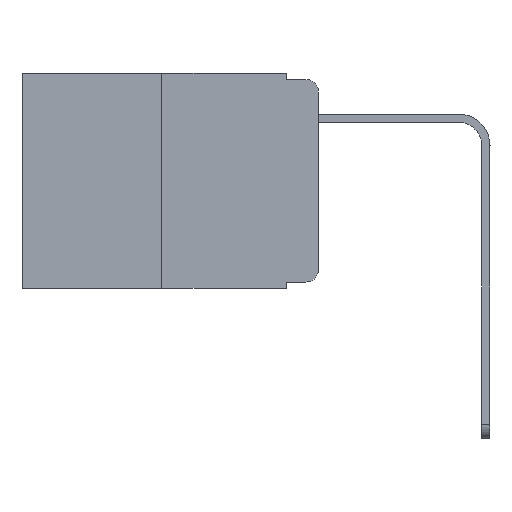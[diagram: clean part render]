
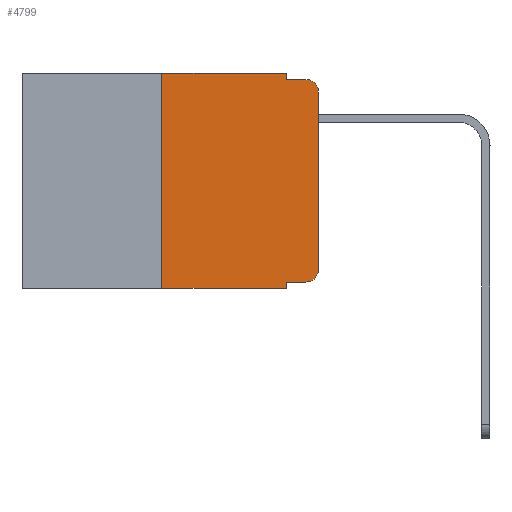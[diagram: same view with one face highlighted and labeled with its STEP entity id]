
A CAD part, left-side view. The second image highlights one B-rep face of the part: STEP entity #4799.
In plain terms, the highlighted planar face has unit normal (-1, 0, 0).
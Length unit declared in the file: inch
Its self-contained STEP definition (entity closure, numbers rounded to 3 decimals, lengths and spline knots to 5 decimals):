
#26 = VECTOR ( 'NONE', #664, 39.37008 ) ;
#181 = LINE ( 'NONE', #2816, #5194 ) ;
#367 = ORIENTED_EDGE ( 'NONE', *, *, #5825, .T. ) ;
#458 = CARTESIAN_POINT ( 'NONE',  ( 0., 0.473, 0. ) ) ;
#626 = EDGE_CURVE ( 'NONE', #7252, #5848, #4277, .T. ) ;
#664 = DIRECTION ( 'NONE',  ( 0., 0., 1. ) ) ;
#673 = CARTESIAN_POINT ( 'NONE',  ( 0., 0.02, -0.03 ) ) ;
#849 = VECTOR ( 'NONE', #5323, 39.37008 ) ;
#954 = ORIENTED_EDGE ( 'NONE', *, *, #626, .F. ) ;
#1013 = VECTOR ( 'NONE', #5104, 39.37008 ) ;
#1018 = VECTOR ( 'NONE', #8433, 39.37008 ) ;
#1101 = LINE ( 'NONE', #2845, #849 ) ;
#1261 = PLANE ( 'NONE',  #10363 ) ;
#1367 = EDGE_CURVE ( 'NONE', #1961, #3718, #2399, .T. ) ;
#1424 = EDGE_CURVE ( 'NONE', #5848, #6477, #9442, .T. ) ;
#1568 = CARTESIAN_POINT ( 'NONE',  ( 0., 0.25, 0. ) ) ;
#1750 = DIRECTION ( 'NONE',  ( 0., -1., 0. ) ) ;
#1810 = CARTESIAN_POINT ( 'NONE',  ( 0., 0.051, -0.01 ) ) ;
#1961 = VERTEX_POINT ( 'NONE', #6617 ) ;
#2343 = VECTOR ( 'NONE', #5141, 39.37008 ) ;
#2399 = LINE ( 'NONE', #1810, #5044 ) ;
#2476 = DIRECTION ( 'NONE',  ( -1., 0., 0. ) ) ;
#2496 = CIRCLE ( 'NONE', #4143, 0.02 ) ;
#2742 = DIRECTION ( 'NONE',  ( 0., 0., -1. ) ) ;
#2808 = CARTESIAN_POINT ( 'NONE',  ( 0., 0.473, 0. ) ) ;
#2816 = CARTESIAN_POINT ( 'NONE',  ( 0., 0.051, 0. ) ) ;
#2845 = CARTESIAN_POINT ( 'NONE',  ( 0., 0.051, -0.333 ) ) ;
#2861 = ORIENTED_EDGE ( 'NONE', *, *, #3949, .F. ) ;
#3322 = ORIENTED_EDGE ( 'NONE', *, *, #5238, .T. ) ;
#3520 = DIRECTION ( 'NONE',  ( 0., 0., -1. ) ) ;
#3547 = CARTESIAN_POINT ( 'NONE',  ( 0., 0., -0.313 ) ) ;
#3718 = VERTEX_POINT ( 'NONE', #6974 ) ;
#3790 = EDGE_CURVE ( 'NONE', #9570, #6513, #1101, .T. ) ;
#3949 = EDGE_CURVE ( 'NONE', #6477, #1961, #10287, .T. ) ;
#4033 = CARTESIAN_POINT ( 'NONE',  ( 0., 0.02, -0.333 ) ) ;
#4143 = AXIS2_PLACEMENT_3D ( 'NONE', #4762, #2476, #7962 ) ;
#4277 = LINE ( 'NONE', #5438, #26 ) ;
#4375 = DIRECTION ( 'NONE',  ( 1., 0., 0. ) ) ;
#4427 = CARTESIAN_POINT ( 'NONE',  ( 0., 0.051, 0. ) ) ;
#4578 = ORIENTED_EDGE ( 'NONE', *, *, #5858, .T. ) ;
#4601 = ORIENTED_EDGE ( 'NONE', *, *, #9212, .F. ) ;
#4762 = CARTESIAN_POINT ( 'NONE',  ( 0., 0.02, -0.313 ) ) ;
#4799 = ADVANCED_FACE ( 'NONE', ( #7553 ), #1261, .F. ) ;
#4835 = VERTEX_POINT ( 'NONE', #6886 ) ;
#5044 = VECTOR ( 'NONE', #1750, 39.37008 ) ;
#5104 = DIRECTION ( 'NONE',  ( 0., -1., 0. ) ) ;
#5141 = DIRECTION ( 'NONE',  ( 0., 0., -1. ) ) ;
#5194 = VECTOR ( 'NONE', #2742, 39.37008 ) ;
#5238 = EDGE_CURVE ( 'NONE', #7252, #4835, #9960, .T. ) ;
#5323 = DIRECTION ( 'NONE',  ( 0., -1., 0. ) ) ;
#5438 = CARTESIAN_POINT ( 'NONE',  ( 0., 0.25, 0. ) ) ;
#5783 = CARTESIAN_POINT ( 'NONE',  ( 0., 0.051, -0.333 ) ) ;
#5825 = EDGE_CURVE ( 'NONE', #7734, #3718, #8567, .T. ) ;
#5848 = VERTEX_POINT ( 'NONE', #1568 ) ;
#5858 = EDGE_CURVE ( 'NONE', #6513, #6209, #2496, .T. ) ;
#6209 = VERTEX_POINT ( 'NONE', #3547 ) ;
#6477 = VERTEX_POINT ( 'NONE', #7918 ) ;
#6513 = VERTEX_POINT ( 'NONE', #4033 ) ;
#6617 = CARTESIAN_POINT ( 'NONE',  ( 0., 0.051, -0.01 ) ) ;
#6745 = CARTESIAN_POINT ( 'NONE',  ( 0., 0., -0.03 ) ) ;
#6886 = CARTESIAN_POINT ( 'NONE',  ( 0., 0.051, -0.343 ) ) ;
#6974 = CARTESIAN_POINT ( 'NONE',  ( 0., 0.02, -0.01 ) ) ;
#7079 = DIRECTION ( 'NONE',  ( -1., 0., 0. ) ) ;
#7128 = EDGE_LOOP ( 'NONE', ( #10034, #367, #8762, #2861, #9351, #954, #3322, #4601, #8982, #4578 ) ) ;
#7252 = VERTEX_POINT ( 'NONE', #10001 ) ;
#7553 = FACE_OUTER_BOUND ( 'NONE', #7128, .T. ) ;
#7734 = VERTEX_POINT ( 'NONE', #6745 ) ;
#7918 = CARTESIAN_POINT ( 'NONE',  ( 0., 0.051, 0. ) ) ;
#7962 = DIRECTION ( 'NONE',  ( 0., 0., -1. ) ) ;
#7964 = VECTOR ( 'NONE', #8838, 39.37008 ) ;
#8433 = DIRECTION ( 'NONE',  ( 0., -1., 0. ) ) ;
#8567 = CIRCLE ( 'NONE', #9026, 0.02 ) ;
#8718 = DIRECTION ( 'NONE',  ( 0., 0., -1. ) ) ;
#8762 = ORIENTED_EDGE ( 'NONE', *, *, #1367, .F. ) ;
#8838 = DIRECTION ( 'NONE',  ( 0., 0., 1. ) ) ;
#8898 = EDGE_CURVE ( 'NONE', #6209, #7734, #9482, .T. ) ;
#8982 = ORIENTED_EDGE ( 'NONE', *, *, #3790, .T. ) ;
#9026 = AXIS2_PLACEMENT_3D ( 'NONE', #673, #7079, #8718 ) ;
#9156 = CARTESIAN_POINT ( 'NONE',  ( 0., 0.473, -0.343 ) ) ;
#9212 = EDGE_CURVE ( 'NONE', #9570, #4835, #181, .T. ) ;
#9351 = ORIENTED_EDGE ( 'NONE', *, *, #1424, .F. ) ;
#9442 = LINE ( 'NONE', #458, #1018 ) ;
#9482 = LINE ( 'NONE', #9534, #7964 ) ;
#9534 = CARTESIAN_POINT ( 'NONE',  ( 0., 0., 0. ) ) ;
#9570 = VERTEX_POINT ( 'NONE', #5783 ) ;
#9960 = LINE ( 'NONE', #9156, #1013 ) ;
#10001 = CARTESIAN_POINT ( 'NONE',  ( 0., 0.25, -0.343 ) ) ;
#10034 = ORIENTED_EDGE ( 'NONE', *, *, #8898, .T. ) ;
#10287 = LINE ( 'NONE', #4427, #2343 ) ;
#10363 = AXIS2_PLACEMENT_3D ( 'NONE', #2808, #4375, #3520 ) ;
